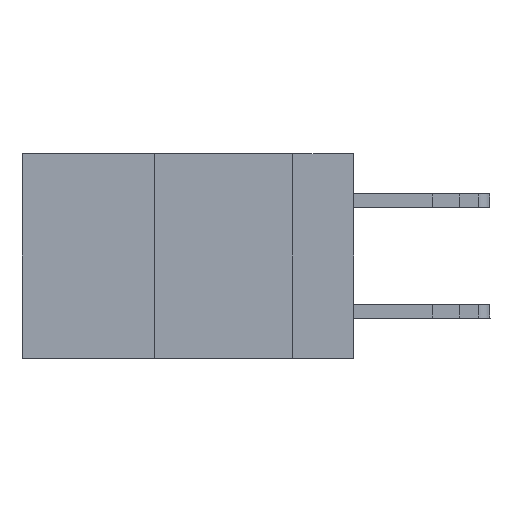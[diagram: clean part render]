
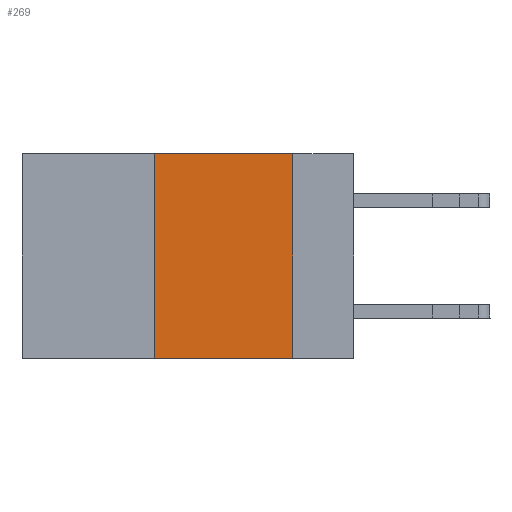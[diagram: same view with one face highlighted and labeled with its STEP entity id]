
A CAD part, left-side view. The second image highlights one B-rep face of the part: STEP entity #269.
In plain terms, the highlighted planar face has unit normal (-1, 0, 0).
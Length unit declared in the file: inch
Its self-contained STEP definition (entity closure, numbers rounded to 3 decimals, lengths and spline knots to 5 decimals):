
#100 = CARTESIAN_POINT ( 'NONE',  ( 0., 0.36, -0.37 ) ) ;
#269 = ADVANCED_FACE ( 'NONE', ( #5858 ), #8623, .F. ) ;
#372 = CARTESIAN_POINT ( 'NONE',  ( 0., 0.6, 0. ) ) ;
#500 = ORIENTED_EDGE ( 'NONE', *, *, #4871, .F. ) ;
#560 = LINE ( 'NONE', #1731, #11432 ) ;
#939 = DIRECTION ( 'NONE',  ( 0., 0., -1. ) ) ;
#1145 = DIRECTION ( 'NONE',  ( 0., -1., 0. ) ) ;
#1731 = CARTESIAN_POINT ( 'NONE',  ( 0., 0.6, 0. ) ) ;
#2025 = CARTESIAN_POINT ( 'NONE',  ( 0., 0.36, 0. ) ) ;
#2183 = VECTOR ( 'NONE', #3539, 39.37008 ) ;
#2988 = CARTESIAN_POINT ( 'NONE',  ( 0., 0.36, 0. ) ) ;
#3181 = ORIENTED_EDGE ( 'NONE', *, *, #15496, .F. ) ;
#3539 = DIRECTION ( 'NONE',  ( 0., 0., -1. ) ) ;
#3749 = CARTESIAN_POINT ( 'NONE',  ( 0., 0.6, -0.37 ) ) ;
#4347 = VERTEX_POINT ( 'NONE', #2988 ) ;
#4766 = DIRECTION ( 'NONE',  ( 0., 0., 1. ) ) ;
#4871 = EDGE_CURVE ( 'NONE', #6771, #12150, #15004, .T. ) ;
#5858 = FACE_OUTER_BOUND ( 'NONE', #14624, .T. ) ;
#5877 = CARTESIAN_POINT ( 'NONE',  ( 0., 0.11, 0. ) ) ;
#6276 = CARTESIAN_POINT ( 'NONE',  ( 0., 0.11, -0.37 ) ) ;
#6640 = EDGE_CURVE ( 'NONE', #7621, #12150, #15204, .T. ) ;
#6771 = VERTEX_POINT ( 'NONE', #11770 ) ;
#6991 = EDGE_CURVE ( 'NONE', #4347, #6771, #560, .T. ) ;
#7621 = VERTEX_POINT ( 'NONE', #100 ) ;
#8332 = AXIS2_PLACEMENT_3D ( 'NONE', #372, #11924, #939 ) ;
#8453 = LINE ( 'NONE', #2025, #9953 ) ;
#8623 = PLANE ( 'NONE',  #8332 ) ;
#9953 = VECTOR ( 'NONE', #4766, 39.37008 ) ;
#11310 = ORIENTED_EDGE ( 'NONE', *, *, #6640, .T. ) ;
#11432 = VECTOR ( 'NONE', #15727, 39.37008 ) ;
#11770 = CARTESIAN_POINT ( 'NONE',  ( 0., 0.11, 0. ) ) ;
#11924 = DIRECTION ( 'NONE',  ( 1., 0., 0. ) ) ;
#12150 = VERTEX_POINT ( 'NONE', #6276 ) ;
#14048 = VECTOR ( 'NONE', #1145, 39.37008 ) ;
#14624 = EDGE_LOOP ( 'NONE', ( #500, #16262, #3181, #11310 ) ) ;
#15004 = LINE ( 'NONE', #5877, #2183 ) ;
#15204 = LINE ( 'NONE', #3749, #14048 ) ;
#15496 = EDGE_CURVE ( 'NONE', #7621, #4347, #8453, .T. ) ;
#15727 = DIRECTION ( 'NONE',  ( 0., -1., 0. ) ) ;
#16262 = ORIENTED_EDGE ( 'NONE', *, *, #6991, .F. ) ;
